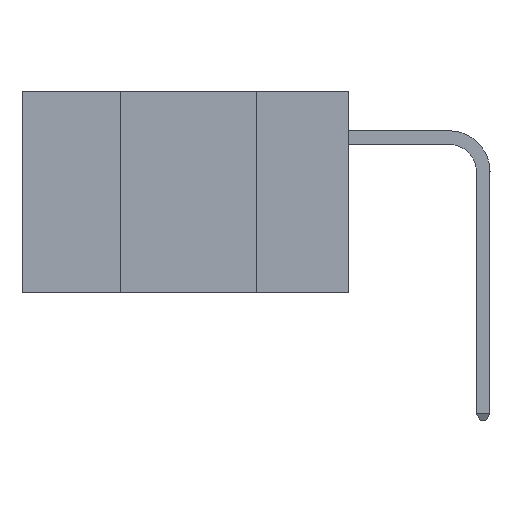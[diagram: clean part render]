
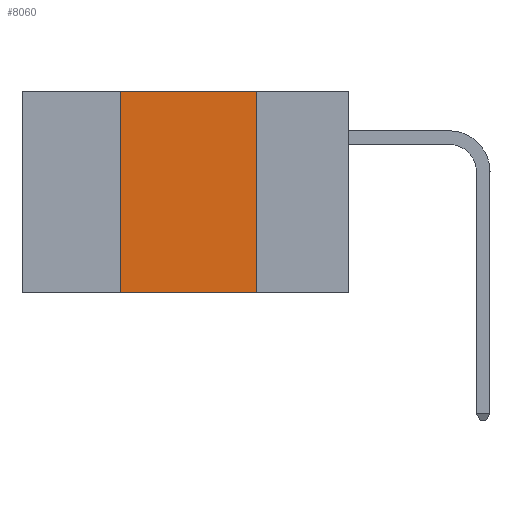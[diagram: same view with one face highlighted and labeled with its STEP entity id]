
A CAD part, left-side view. The second image highlights one B-rep face of the part: STEP entity #8060.
In plain terms, the highlighted planar face has unit normal (-1, 0, 0).
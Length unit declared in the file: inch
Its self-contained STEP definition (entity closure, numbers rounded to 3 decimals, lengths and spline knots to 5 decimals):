
#145 = VERTEX_POINT ( 'NONE', #2865 ) ;
#977 = VERTEX_POINT ( 'NONE', #11041 ) ;
#1605 = CARTESIAN_POINT ( 'NONE',  ( 0., 0.42, 0. ) ) ;
#1992 = ORIENTED_EDGE ( 'NONE', *, *, #13758, .T. ) ;
#2724 = LINE ( 'NONE', #9020, #10232 ) ;
#2821 = DIRECTION ( 'NONE',  ( 0., -1., 0. ) ) ;
#2865 = CARTESIAN_POINT ( 'NONE',  ( 0., 0.17, 0. ) ) ;
#4054 = ORIENTED_EDGE ( 'NONE', *, *, #13457, .F. ) ;
#4119 = ORIENTED_EDGE ( 'NONE', *, *, #15744, .F. ) ;
#5801 = CARTESIAN_POINT ( 'NONE',  ( 0., 0.6, -0.37 ) ) ;
#6124 = EDGE_CURVE ( 'NONE', #7335, #145, #2724, .T. ) ;
#7066 = FACE_OUTER_BOUND ( 'NONE', #12638, .T. ) ;
#7185 = CARTESIAN_POINT ( 'NONE',  ( 0., 0.6, 0. ) ) ;
#7213 = AXIS2_PLACEMENT_3D ( 'NONE', #7185, #8957, #15989 ) ;
#7335 = VERTEX_POINT ( 'NONE', #18234 ) ;
#7679 = DIRECTION ( 'NONE',  ( 0., 0., -1. ) ) ;
#7982 = PLANE ( 'NONE',  #7213 ) ;
#8060 = ADVANCED_FACE ( 'NONE', ( #7066 ), #7982, .F. ) ;
#8957 = DIRECTION ( 'NONE',  ( 1., 0., 0. ) ) ;
#9020 = CARTESIAN_POINT ( 'NONE',  ( 0., 0.6, 0. ) ) ;
#9154 = LINE ( 'NONE', #5801, #17091 ) ;
#10232 = VECTOR ( 'NONE', #10711, 39.37008 ) ;
#10711 = DIRECTION ( 'NONE',  ( 0., -1., 0. ) ) ;
#11041 = CARTESIAN_POINT ( 'NONE',  ( 0., 0.17, -0.37 ) ) ;
#11545 = ORIENTED_EDGE ( 'NONE', *, *, #6124, .F. ) ;
#11704 = LINE ( 'NONE', #1605, #14038 ) ;
#12543 = DIRECTION ( 'NONE',  ( 0., 0., 1. ) ) ;
#12638 = EDGE_LOOP ( 'NONE', ( #4119, #11545, #4054, #1992 ) ) ;
#13291 = LINE ( 'NONE', #13483, #16556 ) ;
#13457 = EDGE_CURVE ( 'NONE', #15780, #7335, #11704, .T. ) ;
#13483 = CARTESIAN_POINT ( 'NONE',  ( 0., 0.17, 0. ) ) ;
#13758 = EDGE_CURVE ( 'NONE', #15780, #977, #9154, .T. ) ;
#14038 = VECTOR ( 'NONE', #12543, 39.37008 ) ;
#14933 = CARTESIAN_POINT ( 'NONE',  ( 0., 0.42, -0.37 ) ) ;
#15744 = EDGE_CURVE ( 'NONE', #145, #977, #13291, .T. ) ;
#15780 = VERTEX_POINT ( 'NONE', #14933 ) ;
#15989 = DIRECTION ( 'NONE',  ( 0., 0., -1. ) ) ;
#16556 = VECTOR ( 'NONE', #7679, 39.37008 ) ;
#17091 = VECTOR ( 'NONE', #2821, 39.37008 ) ;
#18234 = CARTESIAN_POINT ( 'NONE',  ( 0., 0.42, 0. ) ) ;
